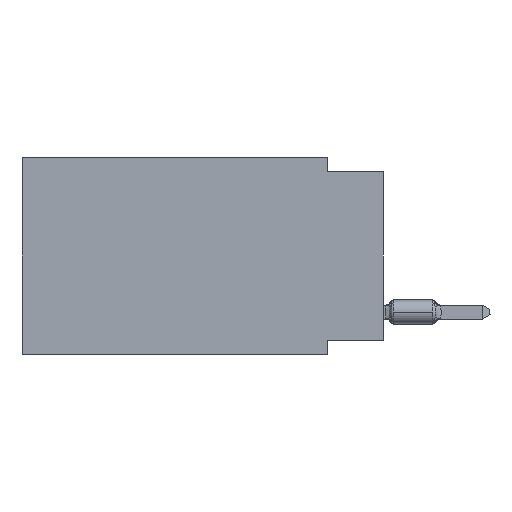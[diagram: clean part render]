
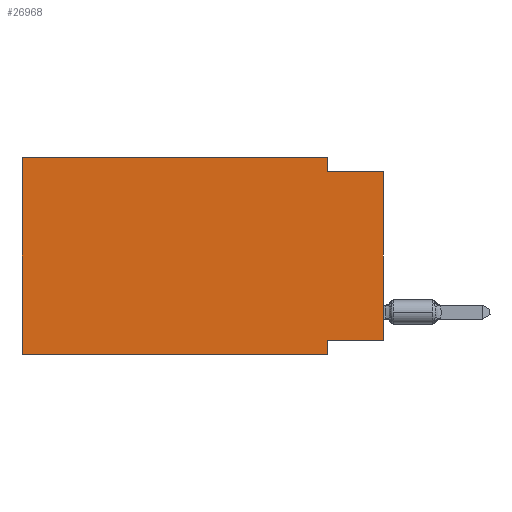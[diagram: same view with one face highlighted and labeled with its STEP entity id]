
A CAD part, left-side view. The second image highlights one B-rep face of the part: STEP entity #26968.
In plain terms, the highlighted planar face has unit normal (-1, 0, 0).
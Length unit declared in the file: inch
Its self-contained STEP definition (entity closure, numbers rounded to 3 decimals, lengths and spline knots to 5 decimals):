
#79 = ORIENTED_EDGE ( 'NONE', *, *, #26324, .F. ) ;
#163 = CARTESIAN_POINT ( 'NONE',  ( 0., 0.645, 0. ) ) ;
#532 = CARTESIAN_POINT ( 'NONE',  ( 0., 0.645, 0. ) ) ;
#1471 = CARTESIAN_POINT ( 'NONE',  ( 0., 0.1, 0. ) ) ;
#1835 = DIRECTION ( 'NONE',  ( 0., -1., 0. ) ) ;
#2499 = CARTESIAN_POINT ( 'NONE',  ( 0., 0.1, -0.35 ) ) ;
#2706 = ORIENTED_EDGE ( 'NONE', *, *, #5258, .F. ) ;
#3153 = VECTOR ( 'NONE', #4337, 39.37008 ) ;
#4059 = CARTESIAN_POINT ( 'NONE',  ( 0., 0., 0. ) ) ;
#4337 = DIRECTION ( 'NONE',  ( 0., 0., 1. ) ) ;
#4734 = ORIENTED_EDGE ( 'NONE', *, *, #10363, .F. ) ;
#4858 = DIRECTION ( 'NONE',  ( 0., 0., 1. ) ) ;
#5258 = EDGE_CURVE ( 'NONE', #21971, #21892, #11214, .T. ) ;
#6932 = LINE ( 'NONE', #25898, #11289 ) ;
#7200 = ORIENTED_EDGE ( 'NONE', *, *, #19546, .T. ) ;
#7215 = CARTESIAN_POINT ( 'NONE',  ( 0., 0., -0.025 ) ) ;
#8632 = VECTOR ( 'NONE', #19646, 39.37008 ) ;
#8784 = VECTOR ( 'NONE', #18692, 39.37008 ) ;
#9066 = CARTESIAN_POINT ( 'NONE',  ( 0., 0.1, -0.025 ) ) ;
#9153 = DIRECTION ( 'NONE',  ( 0., -1., 0. ) ) ;
#9499 = AXIS2_PLACEMENT_3D ( 'NONE', #24445, #13933, #11859 ) ;
#10247 = LINE ( 'NONE', #23127, #8784 ) ;
#10363 = EDGE_CURVE ( 'NONE', #12566, #20575, #22541, .T. ) ;
#10570 = LINE ( 'NONE', #4059, #3153 ) ;
#10751 = VERTEX_POINT ( 'NONE', #24724 ) ;
#11214 = LINE ( 'NONE', #19372, #8632 ) ;
#11261 = EDGE_CURVE ( 'NONE', #21971, #10751, #10570, .T. ) ;
#11289 = VECTOR ( 'NONE', #15387, 39.37008 ) ;
#11443 = FACE_OUTER_BOUND ( 'NONE', #22661, .T. ) ;
#11859 = DIRECTION ( 'NONE',  ( 0., 0., -1. ) ) ;
#12025 = CARTESIAN_POINT ( 'NONE',  ( 0., 0.1, 0. ) ) ;
#12150 = VERTEX_POINT ( 'NONE', #16737 ) ;
#12566 = VERTEX_POINT ( 'NONE', #1471 ) ;
#13282 = EDGE_CURVE ( 'NONE', #26964, #12150, #25888, .T. ) ;
#13933 = DIRECTION ( 'NONE',  ( 1., 0., 0. ) ) ;
#14780 = ORIENTED_EDGE ( 'NONE', *, *, #17002, .F. ) ;
#15387 = DIRECTION ( 'NONE',  ( 0., 0., -1. ) ) ;
#15596 = CARTESIAN_POINT ( 'NONE',  ( 0., 0., -0.325 ) ) ;
#15993 = CARTESIAN_POINT ( 'NONE',  ( 0., 0.645, -0.35 ) ) ;
#16356 = ORIENTED_EDGE ( 'NONE', *, *, #16399, .F. ) ;
#16399 = EDGE_CURVE ( 'NONE', #12150, #12566, #16939, .T. ) ;
#16737 = CARTESIAN_POINT ( 'NONE',  ( 0., 0.645, 0. ) ) ;
#16939 = LINE ( 'NONE', #163, #18498 ) ;
#17002 = EDGE_CURVE ( 'NONE', #20575, #10751, #17868, .T. ) ;
#17868 = LINE ( 'NONE', #7215, #24163 ) ;
#18498 = VECTOR ( 'NONE', #1835, 39.37008 ) ;
#18692 = DIRECTION ( 'NONE',  ( 0., -1., 0. ) ) ;
#18948 = ORIENTED_EDGE ( 'NONE', *, *, #11261, .T. ) ;
#19372 = CARTESIAN_POINT ( 'NONE',  ( 0., 0., -0.325 ) ) ;
#19546 = EDGE_CURVE ( 'NONE', #26964, #26419, #10247, .T. ) ;
#19646 = DIRECTION ( 'NONE',  ( 0., 1., 0. ) ) ;
#19744 = CARTESIAN_POINT ( 'NONE',  ( 0., 0.1, -0.325 ) ) ;
#19867 = PLANE ( 'NONE',  #9499 ) ;
#20575 = VERTEX_POINT ( 'NONE', #9066 ) ;
#21892 = VERTEX_POINT ( 'NONE', #19744 ) ;
#21971 = VERTEX_POINT ( 'NONE', #15596 ) ;
#22541 = LINE ( 'NONE', #12025, #23900 ) ;
#22661 = EDGE_LOOP ( 'NONE', ( #18948, #14780, #4734, #16356, #24082, #7200, #79, #2706 ) ) ;
#22947 = DIRECTION ( 'NONE',  ( 0., 0., -1. ) ) ;
#23127 = CARTESIAN_POINT ( 'NONE',  ( 0., 0.645, -0.35 ) ) ;
#23900 = VECTOR ( 'NONE', #22947, 39.37008 ) ;
#24082 = ORIENTED_EDGE ( 'NONE', *, *, #13282, .F. ) ;
#24163 = VECTOR ( 'NONE', #9153, 39.37008 ) ;
#24445 = CARTESIAN_POINT ( 'NONE',  ( 0., 0.645, 0. ) ) ;
#24724 = CARTESIAN_POINT ( 'NONE',  ( 0., 0., -0.025 ) ) ;
#25757 = VECTOR ( 'NONE', #4858, 39.37008 ) ;
#25888 = LINE ( 'NONE', #532, #25757 ) ;
#25898 = CARTESIAN_POINT ( 'NONE',  ( 0., 0.1, -0.35 ) ) ;
#26324 = EDGE_CURVE ( 'NONE', #21892, #26419, #6932, .T. ) ;
#26419 = VERTEX_POINT ( 'NONE', #2499 ) ;
#26964 = VERTEX_POINT ( 'NONE', #15993 ) ;
#26968 = ADVANCED_FACE ( 'NONE', ( #11443 ), #19867, .F. ) ;
